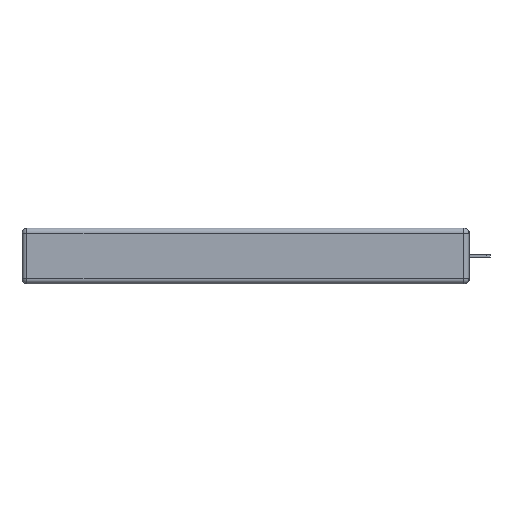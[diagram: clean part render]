
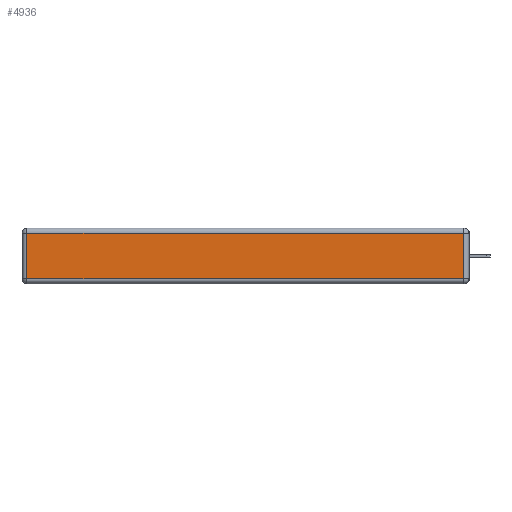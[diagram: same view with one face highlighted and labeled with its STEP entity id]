
A CAD part, left-side view. The second image highlights one B-rep face of the part: STEP entity #4936.
In plain terms, the highlighted planar face has unit normal (-1, 0, 0).
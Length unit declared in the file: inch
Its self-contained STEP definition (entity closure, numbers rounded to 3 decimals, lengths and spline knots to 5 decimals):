
#295 = CARTESIAN_POINT ( 'NONE',  ( 0., 0.03, -0.03 ) ) ;
#1085 = CARTESIAN_POINT ( 'NONE',  ( 0., 0.03, -0.313 ) ) ;
#1515 = DIRECTION ( 'NONE',  ( 0., 0., 1. ) ) ;
#2420 = CARTESIAN_POINT ( 'NONE',  ( 0., 2.72, -0.343 ) ) ;
#2458 = VECTOR ( 'NONE', #7791, 39.37008 ) ;
#2587 = PLANE ( 'NONE',  #11576 ) ;
#2658 = FACE_OUTER_BOUND ( 'NONE', #12176, .T. ) ;
#3010 = ORIENTED_EDGE ( 'NONE', *, *, #11750, .T. ) ;
#3138 = LINE ( 'NONE', #2420, #10616 ) ;
#3330 = ORIENTED_EDGE ( 'NONE', *, *, #3689, .T. ) ;
#3334 = ORIENTED_EDGE ( 'NONE', *, *, #5568, .T. ) ;
#3681 = DIRECTION ( 'NONE',  ( 0., 1., 0. ) ) ;
#3689 = EDGE_CURVE ( 'NONE', #4274, #5087, #12563, .T. ) ;
#3894 = CARTESIAN_POINT ( 'NONE',  ( 0., 2.72, -0.03 ) ) ;
#4124 = VERTEX_POINT ( 'NONE', #1085 ) ;
#4274 = VERTEX_POINT ( 'NONE', #295 ) ;
#4559 = VERTEX_POINT ( 'NONE', #7077 ) ;
#4764 = CARTESIAN_POINT ( 'NONE',  ( 0., 0., -0.343 ) ) ;
#4802 = VECTOR ( 'NONE', #6739, 39.37008 ) ;
#4936 = ADVANCED_FACE ( 'NONE', ( #2658 ), #2587, .T. ) ;
#5087 = VERTEX_POINT ( 'NONE', #3894 ) ;
#5294 = LINE ( 'NONE', #8763, #2458 ) ;
#5568 = EDGE_CURVE ( 'NONE', #4559, #4124, #5294, .T. ) ;
#5967 = EDGE_CURVE ( 'NONE', #5087, #4559, #3138, .T. ) ;
#6739 = DIRECTION ( 'NONE',  ( 0., 0., 1. ) ) ;
#7077 = CARTESIAN_POINT ( 'NONE',  ( 0., 2.72, -0.313 ) ) ;
#7476 = DIRECTION ( 'NONE',  ( 0., 0., -1. ) ) ;
#7661 = DIRECTION ( 'NONE',  ( -1., 0., 0. ) ) ;
#7791 = DIRECTION ( 'NONE',  ( 0., -1., 0. ) ) ;
#8763 = CARTESIAN_POINT ( 'NONE',  ( 0., 0., -0.313 ) ) ;
#9259 = LINE ( 'NONE', #12408, #4802 ) ;
#9541 = CARTESIAN_POINT ( 'NONE',  ( 0., 2.75, -0.03 ) ) ;
#10061 = VECTOR ( 'NONE', #3681, 39.37008 ) ;
#10616 = VECTOR ( 'NONE', #7476, 39.37008 ) ;
#11576 = AXIS2_PLACEMENT_3D ( 'NONE', #4764, #7661, #1515 ) ;
#11750 = EDGE_CURVE ( 'NONE', #4124, #4274, #9259, .T. ) ;
#11802 = ORIENTED_EDGE ( 'NONE', *, *, #5967, .T. ) ;
#12176 = EDGE_LOOP ( 'NONE', ( #3334, #3010, #3330, #11802 ) ) ;
#12408 = CARTESIAN_POINT ( 'NONE',  ( 0., 0.03, -0.343 ) ) ;
#12563 = LINE ( 'NONE', #9541, #10061 ) ;
